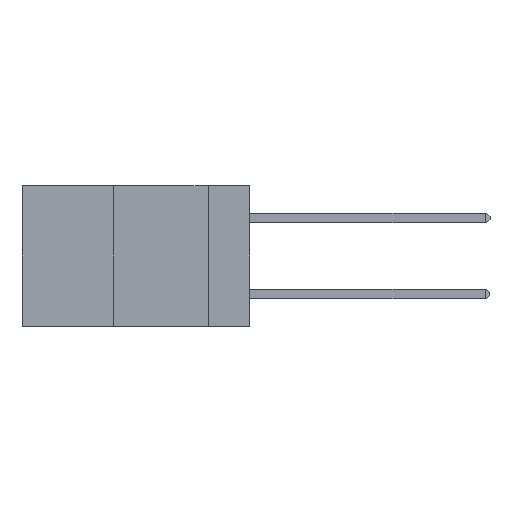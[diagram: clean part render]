
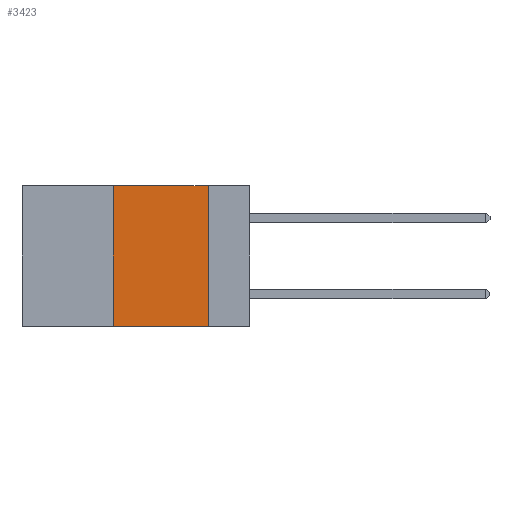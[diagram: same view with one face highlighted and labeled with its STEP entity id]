
A CAD part, left-side view. The second image highlights one B-rep face of the part: STEP entity #3423.
In plain terms, the highlighted planar face has unit normal (-1, 0, 0).
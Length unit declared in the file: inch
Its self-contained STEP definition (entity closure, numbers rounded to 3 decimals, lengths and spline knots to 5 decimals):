
#102 = ORIENTED_EDGE ( 'NONE', *, *, #8899, .T. ) ;
#317 = EDGE_CURVE ( 'NONE', #7990, #9918, #3054, .T. ) ;
#350 = CARTESIAN_POINT ( 'NONE',  ( 0., 0.6, -0.37 ) ) ;
#351 = ORIENTED_EDGE ( 'NONE', *, *, #9152, .F. ) ;
#1275 = DIRECTION ( 'NONE',  ( 0., 0., 1. ) ) ;
#1523 = VERTEX_POINT ( 'NONE', #7084 ) ;
#1809 = CARTESIAN_POINT ( 'NONE',  ( 0., 0.6, 0. ) ) ;
#1948 = LINE ( 'NONE', #350, #10243 ) ;
#2163 = DIRECTION ( 'NONE',  ( 0., 0., -1. ) ) ;
#2168 = FACE_OUTER_BOUND ( 'NONE', #4023, .T. ) ;
#2266 = ORIENTED_EDGE ( 'NONE', *, *, #2751, .F. ) ;
#2305 = CARTESIAN_POINT ( 'NONE',  ( 0., 0.36, 0. ) ) ;
#2629 = ORIENTED_EDGE ( 'NONE', *, *, #317, .F. ) ;
#2751 = EDGE_CURVE ( 'NONE', #1523, #9142, #7089, .T. ) ;
#3054 = LINE ( 'NONE', #2305, #10674 ) ;
#3423 = ADVANCED_FACE ( 'NONE', ( #2168 ), #5116, .F. ) ;
#4023 = EDGE_LOOP ( 'NONE', ( #2266, #351, #2629, #102 ) ) ;
#4836 = CARTESIAN_POINT ( 'NONE',  ( 0., 0.11, -0.37 ) ) ;
#5116 = PLANE ( 'NONE',  #11599 ) ;
#5151 = DIRECTION ( 'NONE',  ( 0., 0., -1. ) ) ;
#6455 = DIRECTION ( 'NONE',  ( 0., -1., 0. ) ) ;
#6778 = VECTOR ( 'NONE', #2163, 39.37008 ) ;
#6848 = LINE ( 'NONE', #1809, #11983 ) ;
#7084 = CARTESIAN_POINT ( 'NONE',  ( 0., 0.11, 0. ) ) ;
#7089 = LINE ( 'NONE', #10159, #6778 ) ;
#7862 = DIRECTION ( 'NONE',  ( 0., -1., 0. ) ) ;
#7990 = VERTEX_POINT ( 'NONE', #12592 ) ;
#8899 = EDGE_CURVE ( 'NONE', #7990, #9142, #1948, .T. ) ;
#9142 = VERTEX_POINT ( 'NONE', #4836 ) ;
#9152 = EDGE_CURVE ( 'NONE', #9918, #1523, #6848, .T. ) ;
#9918 = VERTEX_POINT ( 'NONE', #9971 ) ;
#9971 = CARTESIAN_POINT ( 'NONE',  ( 0., 0.36, 0. ) ) ;
#10099 = CARTESIAN_POINT ( 'NONE',  ( 0., 0.6, 0. ) ) ;
#10159 = CARTESIAN_POINT ( 'NONE',  ( 0., 0.11, 0. ) ) ;
#10243 = VECTOR ( 'NONE', #6455, 39.37008 ) ;
#10674 = VECTOR ( 'NONE', #1275, 39.37008 ) ;
#11044 = DIRECTION ( 'NONE',  ( 1., 0., 0. ) ) ;
#11599 = AXIS2_PLACEMENT_3D ( 'NONE', #10099, #11044, #5151 ) ;
#11983 = VECTOR ( 'NONE', #7862, 39.37008 ) ;
#12592 = CARTESIAN_POINT ( 'NONE',  ( 0., 0.36, -0.37 ) ) ;
